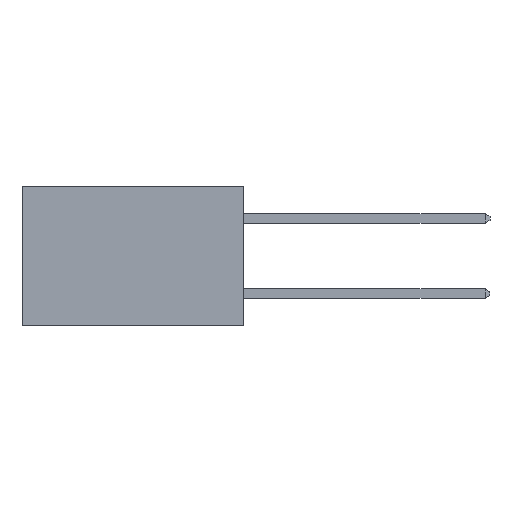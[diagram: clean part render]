
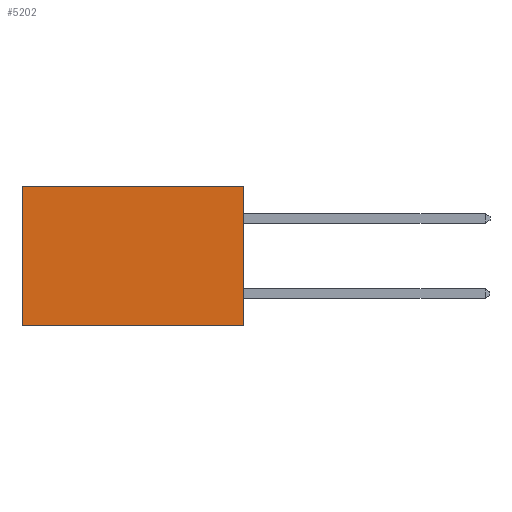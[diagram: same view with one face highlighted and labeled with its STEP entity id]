
A CAD part, left-side view. The second image highlights one B-rep face of the part: STEP entity #5202.
In plain terms, the highlighted planar face has unit normal (-1, 0, 0).
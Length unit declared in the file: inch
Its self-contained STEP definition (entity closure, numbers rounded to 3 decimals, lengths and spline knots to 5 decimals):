
#25 = VERTEX_POINT ( 'NONE', #8319 ) ;
#308 = VECTOR ( 'NONE', #3467, 39.37008 ) ;
#773 = LINE ( 'NONE', #6677, #308 ) ;
#886 = LINE ( 'NONE', #3536, #4912 ) ;
#963 = CARTESIAN_POINT ( 'NONE',  ( 0.277, 0.59, -0.37 ) ) ;
#1169 = DIRECTION ( 'NONE',  ( 1., 0., 0. ) ) ;
#1344 = CARTESIAN_POINT ( 'NONE',  ( 0.277, 0., -0.37 ) ) ;
#1467 = DIRECTION ( 'NONE',  ( 0., 0., -1. ) ) ;
#1642 = LINE ( 'NONE', #7100, #9601 ) ;
#2305 = EDGE_CURVE ( 'NONE', #25, #5438, #773, .T. ) ;
#2381 = VERTEX_POINT ( 'NONE', #5949 ) ;
#3467 = DIRECTION ( 'NONE',  ( 0., 1., 0. ) ) ;
#3468 = DIRECTION ( 'NONE',  ( 0., 1., 0. ) ) ;
#3536 = CARTESIAN_POINT ( 'NONE',  ( 0.277, 0., 0. ) ) ;
#3778 = FACE_OUTER_BOUND ( 'NONE', #8851, .T. ) ;
#4174 = CARTESIAN_POINT ( 'NONE',  ( 0.277, 0.59, -0.37 ) ) ;
#4562 = ORIENTED_EDGE ( 'NONE', *, *, #2305, .F. ) ;
#4868 = ORIENTED_EDGE ( 'NONE', *, *, #5450, .F. ) ;
#4912 = VECTOR ( 'NONE', #3468, 39.37008 ) ;
#5202 = ADVANCED_FACE ( 'NONE', ( #3778 ), #7973, .F. ) ;
#5348 = AXIS2_PLACEMENT_3D ( 'NONE', #1344, #1169, #1467 ) ;
#5438 = VERTEX_POINT ( 'NONE', #4174 ) ;
#5440 = ORIENTED_EDGE ( 'NONE', *, *, #7285, .T. ) ;
#5450 = EDGE_CURVE ( 'NONE', #7596, #25, #1642, .T. ) ;
#5949 = CARTESIAN_POINT ( 'NONE',  ( 0.277, 0.59, 0. ) ) ;
#6665 = ORIENTED_EDGE ( 'NONE', *, *, #8082, .T. ) ;
#6677 = CARTESIAN_POINT ( 'NONE',  ( 0.277, 0., -0.37 ) ) ;
#7100 = CARTESIAN_POINT ( 'NONE',  ( 0.277, 0., -0.37 ) ) ;
#7111 = CARTESIAN_POINT ( 'NONE',  ( 0.277, 0., 0. ) ) ;
#7285 = EDGE_CURVE ( 'NONE', #2381, #5438, #7672, .T. ) ;
#7596 = VERTEX_POINT ( 'NONE', #7111 ) ;
#7657 = DIRECTION ( 'NONE',  ( 0., 0., -1. ) ) ;
#7672 = LINE ( 'NONE', #963, #9562 ) ;
#7973 = PLANE ( 'NONE',  #5348 ) ;
#8082 = EDGE_CURVE ( 'NONE', #7596, #2381, #886, .T. ) ;
#8319 = CARTESIAN_POINT ( 'NONE',  ( 0.277, 0., -0.37 ) ) ;
#8851 = EDGE_LOOP ( 'NONE', ( #5440, #4562, #4868, #6665 ) ) ;
#9562 = VECTOR ( 'NONE', #9671, 39.37008 ) ;
#9601 = VECTOR ( 'NONE', #7657, 39.37008 ) ;
#9671 = DIRECTION ( 'NONE',  ( 0., 0., -1. ) ) ;
